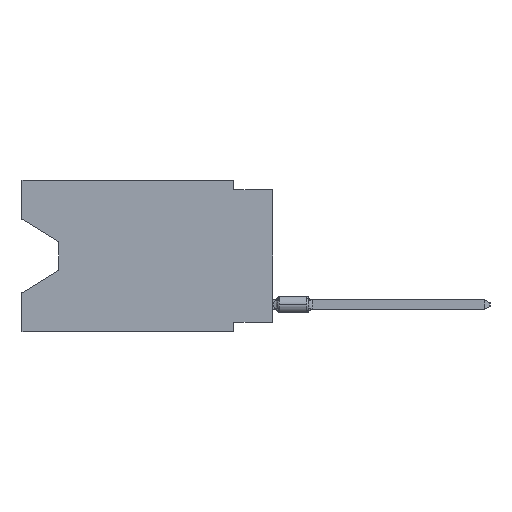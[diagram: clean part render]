
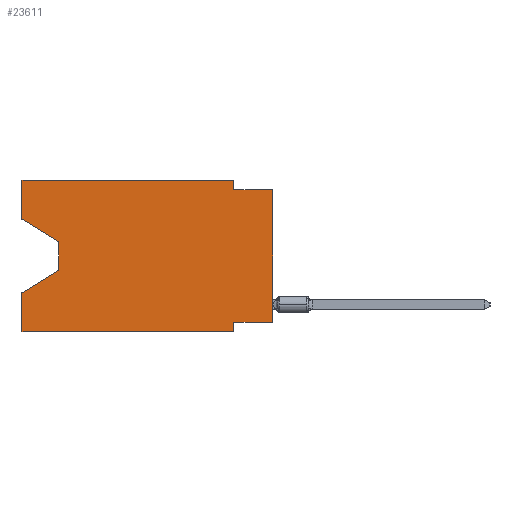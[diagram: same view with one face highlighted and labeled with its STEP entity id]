
A CAD part, left-side view. The second image highlights one B-rep face of the part: STEP entity #23611.
In plain terms, the highlighted planar face has unit normal (-1, 0, 0).
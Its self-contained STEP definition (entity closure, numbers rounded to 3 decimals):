
#148 = ORIENTED_EDGE ( 'NONE', *, *, #32207, .F. ) ;
#341 = VERTEX_POINT ( 'NONE', #4811 ) ;
#414 = ORIENTED_EDGE ( 'NONE', *, *, #8964, .F. ) ;
#613 = LINE ( 'NONE', #8860, #22234 ) ;
#1757 = LINE ( 'NONE', #10548, #19430 ) ;
#2677 = VERTEX_POINT ( 'NONE', #35282 ) ;
#2737 = CARTESIAN_POINT ( 'NONE',  ( 0., 16.383, 0. ) ) ;
#3365 = EDGE_CURVE ( 'NONE', #23897, #4435, #27130, .T. ) ;
#3473 = CARTESIAN_POINT ( 'NONE',  ( 0., 16.383, 0. ) ) ;
#3657 = DIRECTION ( 'NONE',  ( 1., 0., 0. ) ) ;
#3916 = CARTESIAN_POINT ( 'NONE',  ( 0., 0., 0. ) ) ;
#4435 = VERTEX_POINT ( 'NONE', #10422 ) ;
#4568 = EDGE_LOOP ( 'NONE', ( #33250, #16436, #13796, #14400, #15982, #26201, #24578, #16990, #148, #14436, #414, #30527 ) ) ;
#4811 = CARTESIAN_POINT ( 'NONE',  ( 0., 0., -9.271 ) ) ;
#4911 = DIRECTION ( 'NONE',  ( 0., 0., 1. ) ) ;
#6093 = DIRECTION ( 'NONE',  ( 0., -1., 0. ) ) ;
#6412 = DIRECTION ( 'NONE',  ( 0., 0., 1. ) ) ;
#6704 = CARTESIAN_POINT ( 'NONE',  ( 0., 0., -9.271 ) ) ;
#8860 = CARTESIAN_POINT ( 'NONE',  ( 0., 13.97, -4.013 ) ) ;
#8964 = EDGE_CURVE ( 'NONE', #17130, #26854, #25535, .T. ) ;
#9063 = VERTEX_POINT ( 'NONE', #33586 ) ;
#9188 = LINE ( 'NONE', #28364, #32062 ) ;
#9872 = VECTOR ( 'NONE', #24041, 1000. ) ;
#10143 = LINE ( 'NONE', #3916, #21555 ) ;
#10225 = CARTESIAN_POINT ( 'NONE',  ( 0., 2.54, -9.906 ) ) ;
#10228 = LINE ( 'NONE', #24434, #13619 ) ;
#10422 = CARTESIAN_POINT ( 'NONE',  ( 0., 16.383, -7.36 ) ) ;
#10548 = CARTESIAN_POINT ( 'NONE',  ( 0., 2.54, 0. ) ) ;
#10673 = EDGE_CURVE ( 'NONE', #9063, #4435, #29223, .T. ) ;
#11119 = CARTESIAN_POINT ( 'NONE',  ( 0., 13.97, -5.893 ) ) ;
#11656 = DIRECTION ( 'NONE',  ( 0., 0., 1. ) ) ;
#11757 = DIRECTION ( 'NONE',  ( 0., -0.855, -0.519 ) ) ;
#11785 = DIRECTION ( 'NONE',  ( 0., 0., -1. ) ) ;
#11815 = EDGE_CURVE ( 'NONE', #22640, #34694, #32767, .T. ) ;
#11893 = FACE_OUTER_BOUND ( 'NONE', #4568, .T. ) ;
#12067 = PLANE ( 'NONE',  #22714 ) ;
#13434 = EDGE_CURVE ( 'NONE', #9063, #34694, #15188, .T. ) ;
#13619 = VECTOR ( 'NONE', #4911, 1000. ) ;
#13796 = ORIENTED_EDGE ( 'NONE', *, *, #3365, .T. ) ;
#14400 = ORIENTED_EDGE ( 'NONE', *, *, #10673, .F. ) ;
#14436 = ORIENTED_EDGE ( 'NONE', *, *, #19564, .F. ) ;
#15188 = LINE ( 'NONE', #23935, #28532 ) ;
#15349 = DIRECTION ( 'NONE',  ( 0., 0., -1. ) ) ;
#15634 = CARTESIAN_POINT ( 'NONE',  ( 0., 2.54, -9.906 ) ) ;
#15653 = LINE ( 'NONE', #6704, #9872 ) ;
#15982 = ORIENTED_EDGE ( 'NONE', *, *, #13434, .T. ) ;
#16320 = CARTESIAN_POINT ( 'NONE',  ( 0., 13.97, -4.013 ) ) ;
#16436 = ORIENTED_EDGE ( 'NONE', *, *, #25654, .T. ) ;
#16701 = LINE ( 'NONE', #33646, #28586 ) ;
#16990 = ORIENTED_EDGE ( 'NONE', *, *, #24033, .T. ) ;
#17130 = VERTEX_POINT ( 'NONE', #21322 ) ;
#17179 = DIRECTION ( 'NONE',  ( 0., -1., 0. ) ) ;
#17225 = VECTOR ( 'NONE', #18204, 1000. ) ;
#17659 = CARTESIAN_POINT ( 'NONE',  ( 0., 2.54, -0.635 ) ) ;
#18204 = DIRECTION ( 'NONE',  ( 0., 0.855, -0.519 ) ) ;
#18407 = DIRECTION ( 'NONE',  ( 0., 0., -1. ) ) ;
#19272 = DIRECTION ( 'NONE',  ( 0., 0., -1. ) ) ;
#19430 = VECTOR ( 'NONE', #18407, 1000. ) ;
#19564 = EDGE_CURVE ( 'NONE', #26854, #29147, #1757, .T. ) ;
#21322 = CARTESIAN_POINT ( 'NONE',  ( 0., 16.383, 0. ) ) ;
#21493 = EDGE_CURVE ( 'NONE', #29926, #17130, #10228, .T. ) ;
#21555 = VECTOR ( 'NONE', #11656, 1000. ) ;
#22234 = VECTOR ( 'NONE', #11785, 1000. ) ;
#22640 = VERTEX_POINT ( 'NONE', #34361 ) ;
#22714 = AXIS2_PLACEMENT_3D ( 'NONE', #3473, #3657, #15349 ) ;
#23611 = ADVANCED_FACE ( 'NONE', ( #11893 ), #12067, .F. ) ;
#23897 = VERTEX_POINT ( 'NONE', #11119 ) ;
#23935 = CARTESIAN_POINT ( 'NONE',  ( 0., 16.383, -9.906 ) ) ;
#24033 = EDGE_CURVE ( 'NONE', #341, #2677, #10143, .T. ) ;
#24041 = DIRECTION ( 'NONE',  ( 0., 1., 0. ) ) ;
#24259 = EDGE_CURVE ( 'NONE', #29926, #30891, #9188, .T. ) ;
#24434 = CARTESIAN_POINT ( 'NONE',  ( 0., 16.383, 0. ) ) ;
#24578 = ORIENTED_EDGE ( 'NONE', *, *, #28160, .F. ) ;
#24783 = VECTOR ( 'NONE', #17179, 1000. ) ;
#25535 = LINE ( 'NONE', #2737, #24783 ) ;
#25654 = EDGE_CURVE ( 'NONE', #30891, #23897, #613, .T. ) ;
#26201 = ORIENTED_EDGE ( 'NONE', *, *, #11815, .F. ) ;
#26364 = CARTESIAN_POINT ( 'NONE',  ( 0., 2.54, 0. ) ) ;
#26854 = VERTEX_POINT ( 'NONE', #26364 ) ;
#27130 = LINE ( 'NONE', #31883, #17225 ) ;
#28160 = EDGE_CURVE ( 'NONE', #341, #22640, #15653, .T. ) ;
#28364 = CARTESIAN_POINT ( 'NONE',  ( 0., 16.383, -2.546 ) ) ;
#28532 = VECTOR ( 'NONE', #31960, 1000. ) ;
#28586 = VECTOR ( 'NONE', #6093, 1000. ) ;
#28835 = CARTESIAN_POINT ( 'NONE',  ( 0., 16.383, -2.546 ) ) ;
#29147 = VERTEX_POINT ( 'NONE', #17659 ) ;
#29223 = LINE ( 'NONE', #31420, #29321 ) ;
#29321 = VECTOR ( 'NONE', #6412, 1000. ) ;
#29926 = VERTEX_POINT ( 'NONE', #28835 ) ;
#30527 = ORIENTED_EDGE ( 'NONE', *, *, #21493, .F. ) ;
#30891 = VERTEX_POINT ( 'NONE', #16320 ) ;
#31420 = CARTESIAN_POINT ( 'NONE',  ( 0., 16.383, 0. ) ) ;
#31602 = VECTOR ( 'NONE', #19272, 1000. ) ;
#31883 = CARTESIAN_POINT ( 'NONE',  ( 0., 13.97, -5.893 ) ) ;
#31960 = DIRECTION ( 'NONE',  ( 0., -1., 0. ) ) ;
#32062 = VECTOR ( 'NONE', #11757, 1000. ) ;
#32207 = EDGE_CURVE ( 'NONE', #29147, #2677, #16701, .T. ) ;
#32767 = LINE ( 'NONE', #15634, #31602 ) ;
#33250 = ORIENTED_EDGE ( 'NONE', *, *, #24259, .T. ) ;
#33586 = CARTESIAN_POINT ( 'NONE',  ( 0., 16.383, -9.906 ) ) ;
#33646 = CARTESIAN_POINT ( 'NONE',  ( 0., 0., -0.635 ) ) ;
#34361 = CARTESIAN_POINT ( 'NONE',  ( 0., 2.54, -9.271 ) ) ;
#34694 = VERTEX_POINT ( 'NONE', #10225 ) ;
#35282 = CARTESIAN_POINT ( 'NONE',  ( 0., 0., -0.635 ) ) ;
